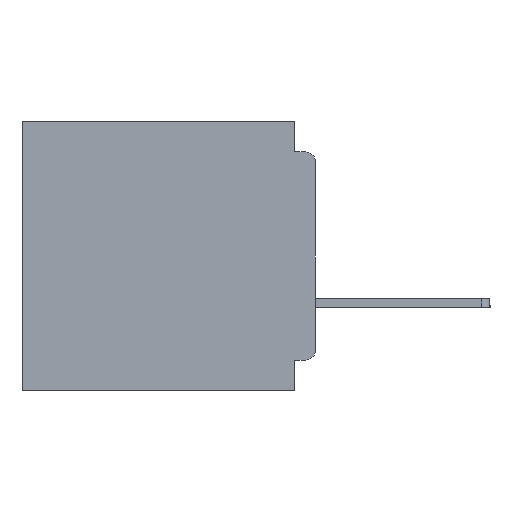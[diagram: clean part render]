
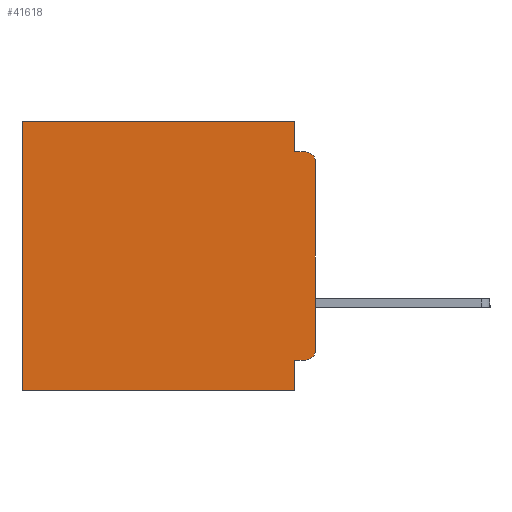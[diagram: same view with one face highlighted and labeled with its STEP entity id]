
A CAD part, left-side view. The second image highlights one B-rep face of the part: STEP entity #41618.
In plain terms, the highlighted planar face has unit normal (-1, 0, 0).
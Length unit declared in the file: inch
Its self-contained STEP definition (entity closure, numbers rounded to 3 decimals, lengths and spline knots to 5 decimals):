
#2446 = CARTESIAN_POINT ( 'NONE',  ( 0.3, 0.031, -0.4 ) ) ;
#2612 = CARTESIAN_POINT ( 'NONE',  ( 0.3, 0.015, -0.06 ) ) ;
#3171 = VERTEX_POINT ( 'NONE', #22335 ) ;
#6234 = CARTESIAN_POINT ( 'NONE',  ( 0.3, 0., -0.4 ) ) ;
#6388 = VERTEX_POINT ( 'NONE', #48988 ) ;
#7366 = DIRECTION ( 'NONE',  ( 0., 0., -1. ) ) ;
#7890 = DIRECTION ( 'NONE',  ( 0., 0., -1. ) ) ;
#9146 = CIRCLE ( 'NONE', #24740, 0.015 ) ;
#9565 = DIRECTION ( 'NONE',  ( 0., 0., -1. ) ) ;
#11077 = VECTOR ( 'NONE', #46080, 39.37008 ) ;
#11218 = DIRECTION ( 'NONE',  ( 0., -1., 0. ) ) ;
#11946 = LINE ( 'NONE', #33048, #47137 ) ;
#11952 = EDGE_CURVE ( 'NONE', #30338, #41653, #30429, .T. ) ;
#12110 = ORIENTED_EDGE ( 'NONE', *, *, #29210, .T. ) ;
#13073 = EDGE_CURVE ( 'NONE', #29207, #38193, #18975, .T. ) ;
#13582 = VERTEX_POINT ( 'NONE', #2446 ) ;
#13674 = LINE ( 'NONE', #46692, #27414 ) ;
#15145 = CARTESIAN_POINT ( 'NONE',  ( 0.3, 0., -0.4 ) ) ;
#15615 = PLANE ( 'NONE',  #29281 ) ;
#17244 = EDGE_CURVE ( 'NONE', #41653, #31601, #52056, .T. ) ;
#17303 = CARTESIAN_POINT ( 'NONE',  ( 0.3, 0., -0.4 ) ) ;
#17376 = ORIENTED_EDGE ( 'NONE', *, *, #46938, .F. ) ;
#18975 = LINE ( 'NONE', #21887, #32690 ) ;
#19885 = CARTESIAN_POINT ( 'NONE',  ( 0.3, 0.015, -0.34 ) ) ;
#20025 = LINE ( 'NONE', #17303, #30853 ) ;
#20258 = DIRECTION ( 'NONE',  ( 1., 0., 0. ) ) ;
#20322 = ORIENTED_EDGE ( 'NONE', *, *, #34973, .T. ) ;
#21071 = EDGE_CURVE ( 'NONE', #55780, #6388, #9146, .T. ) ;
#21154 = CARTESIAN_POINT ( 'NONE',  ( 0.3, 0.437, 0. ) ) ;
#21887 = CARTESIAN_POINT ( 'NONE',  ( 0.3, 0.437, -0.4 ) ) ;
#21986 = DIRECTION ( 'NONE',  ( 0., 1., 0. ) ) ;
#22335 = CARTESIAN_POINT ( 'NONE',  ( 0.3, 0.031, -0.355 ) ) ;
#24586 = DIRECTION ( 'NONE',  ( 0., 0., -1. ) ) ;
#24740 = AXIS2_PLACEMENT_3D ( 'NONE', #19885, #51866, #24586 ) ;
#24998 = EDGE_CURVE ( 'NONE', #55780, #3171, #13674, .T. ) ;
#25134 = CARTESIAN_POINT ( 'NONE',  ( 0.3, 0.031, -0.045 ) ) ;
#25975 = EDGE_CURVE ( 'NONE', #13582, #38193, #20025, .T. ) ;
#26656 = EDGE_CURVE ( 'NONE', #27435, #6388, #43479, .T. ) ;
#27414 = VECTOR ( 'NONE', #46298, 39.37008 ) ;
#27435 = VERTEX_POINT ( 'NONE', #53884 ) ;
#27922 = ORIENTED_EDGE ( 'NONE', *, *, #11952, .F. ) ;
#29207 = VERTEX_POINT ( 'NONE', #21154 ) ;
#29210 = EDGE_CURVE ( 'NONE', #27435, #31601, #51880, .T. ) ;
#29281 = AXIS2_PLACEMENT_3D ( 'NONE', #6234, #20258, #52214 ) ;
#29565 = ORIENTED_EDGE ( 'NONE', *, *, #13073, .T. ) ;
#29863 = EDGE_LOOP ( 'NONE', ( #57712, #12110, #33019, #27922, #20322, #29565, #46485, #17376, #41854, #46655 ) ) ;
#30338 = VERTEX_POINT ( 'NONE', #35894 ) ;
#30429 = LINE ( 'NONE', #37167, #39664 ) ;
#30853 = VECTOR ( 'NONE', #21986, 39.37008 ) ;
#31601 = VERTEX_POINT ( 'NONE', #46127 ) ;
#32690 = VECTOR ( 'NONE', #7890, 39.37008 ) ;
#33019 = ORIENTED_EDGE ( 'NONE', *, *, #17244, .F. ) ;
#33048 = CARTESIAN_POINT ( 'NONE',  ( 0.3, 0.031, -0.4 ) ) ;
#33622 = CARTESIAN_POINT ( 'NONE',  ( 0.3, 0.437, -0.4 ) ) ;
#33746 = CARTESIAN_POINT ( 'NONE',  ( 0.3, 0.015, -0.355 ) ) ;
#33824 = AXIS2_PLACEMENT_3D ( 'NONE', #2612, #35025, #7366 ) ;
#34237 = CARTESIAN_POINT ( 'NONE',  ( 0.3, 0., -0.045 ) ) ;
#34973 = EDGE_CURVE ( 'NONE', #30338, #29207, #49140, .T. ) ;
#35025 = DIRECTION ( 'NONE',  ( -1., 0., 0. ) ) ;
#35894 = CARTESIAN_POINT ( 'NONE',  ( 0.3, 0.031, 0. ) ) ;
#36902 = CARTESIAN_POINT ( 'NONE',  ( 0.3, 0., 0. ) ) ;
#37167 = CARTESIAN_POINT ( 'NONE',  ( 0.3, 0.031, 0. ) ) ;
#38193 = VERTEX_POINT ( 'NONE', #33622 ) ;
#39664 = VECTOR ( 'NONE', #9565, 39.37008 ) ;
#39952 = VECTOR ( 'NONE', #11218, 39.37008 ) ;
#41618 = ADVANCED_FACE ( 'NONE', ( #44756 ), #15615, .F. ) ;
#41653 = VERTEX_POINT ( 'NONE', #25134 ) ;
#41854 = ORIENTED_EDGE ( 'NONE', *, *, #24998, .F. ) ;
#43479 = LINE ( 'NONE', #15145, #54078 ) ;
#44756 = FACE_OUTER_BOUND ( 'NONE', #29863, .T. ) ;
#46080 = DIRECTION ( 'NONE',  ( 0., 1., 0. ) ) ;
#46127 = CARTESIAN_POINT ( 'NONE',  ( 0.3, 0.015, -0.045 ) ) ;
#46298 = DIRECTION ( 'NONE',  ( 0., 1., 0. ) ) ;
#46485 = ORIENTED_EDGE ( 'NONE', *, *, #25975, .F. ) ;
#46655 = ORIENTED_EDGE ( 'NONE', *, *, #21071, .T. ) ;
#46692 = CARTESIAN_POINT ( 'NONE',  ( 0.3, 0., -0.355 ) ) ;
#46938 = EDGE_CURVE ( 'NONE', #3171, #13582, #11946, .T. ) ;
#47137 = VECTOR ( 'NONE', #51340, 39.37008 ) ;
#48988 = CARTESIAN_POINT ( 'NONE',  ( 0.3, 0., -0.34 ) ) ;
#49140 = LINE ( 'NONE', #36902, #11077 ) ;
#51340 = DIRECTION ( 'NONE',  ( 0., 0., -1. ) ) ;
#51754 = DIRECTION ( 'NONE',  ( 0., 0., -1. ) ) ;
#51866 = DIRECTION ( 'NONE',  ( -1., 0., 0. ) ) ;
#51880 = CIRCLE ( 'NONE', #33824, 0.015 ) ;
#52056 = LINE ( 'NONE', #34237, #39952 ) ;
#52214 = DIRECTION ( 'NONE',  ( 0., 0., -1. ) ) ;
#53884 = CARTESIAN_POINT ( 'NONE',  ( 0.3, 0., -0.06 ) ) ;
#54078 = VECTOR ( 'NONE', #51754, 39.37008 ) ;
#55780 = VERTEX_POINT ( 'NONE', #33746 ) ;
#57712 = ORIENTED_EDGE ( 'NONE', *, *, #26656, .F. ) ;
